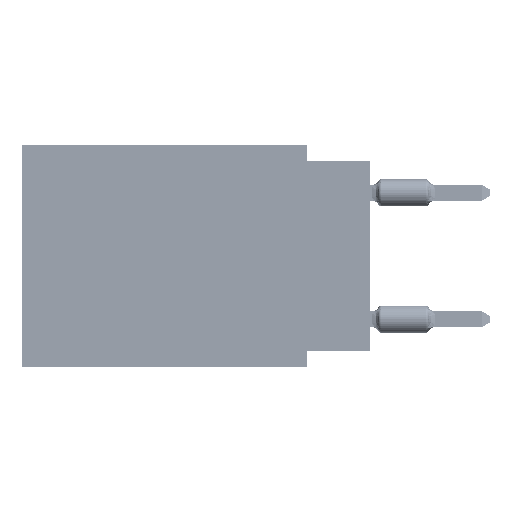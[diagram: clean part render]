
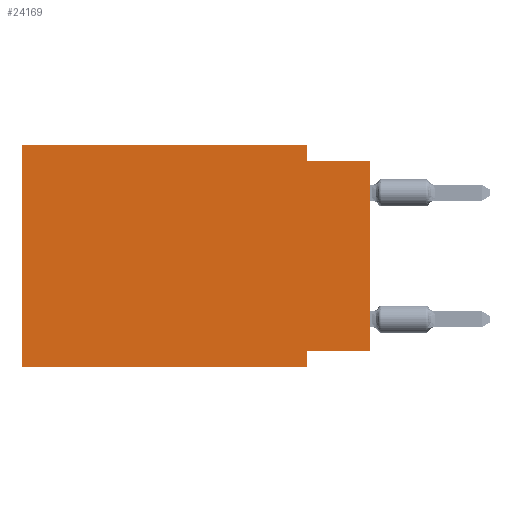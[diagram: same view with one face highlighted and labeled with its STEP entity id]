
A CAD part, left-side view. The second image highlights one B-rep face of the part: STEP entity #24169.
In plain terms, the highlighted planar face has unit normal (-1, 0, 0).
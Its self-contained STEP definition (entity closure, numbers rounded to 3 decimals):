
#1095 = DIRECTION ( 'NONE',  ( 0., 0., -1. ) ) ;
#3180 = CARTESIAN_POINT ( 'NONE',  ( 0., 2.54, 0. ) ) ;
#3432 = DIRECTION ( 'NONE',  ( 0., 0., 1. ) ) ;
#3450 = EDGE_CURVE ( 'NONE', #73395, #56345, #50145, .T. ) ;
#3740 = LINE ( 'NONE', #25478, #61603 ) ;
#6093 = ORIENTED_EDGE ( 'NONE', *, *, #75973, .F. ) ;
#7841 = DIRECTION ( 'NONE',  ( 1., 0., 0. ) ) ;
#11093 = EDGE_CURVE ( 'NONE', #56331, #86210, #3740, .T. ) ;
#12605 = CARTESIAN_POINT ( 'NONE',  ( 0., 0., -0.635 ) ) ;
#15490 = CARTESIAN_POINT ( 'NONE',  ( 0., 2.54, 0. ) ) ;
#16771 = ORIENTED_EDGE ( 'NONE', *, *, #11093, .F. ) ;
#18758 = ORIENTED_EDGE ( 'NONE', *, *, #63439, .F. ) ;
#19653 = LINE ( 'NONE', #64535, #55077 ) ;
#21653 = CARTESIAN_POINT ( 'NONE',  ( 0., 0., -8.255 ) ) ;
#21686 = VERTEX_POINT ( 'NONE', #22330 ) ;
#22330 = CARTESIAN_POINT ( 'NONE',  ( 0., 0., -0.635 ) ) ;
#22955 = LINE ( 'NONE', #95357, #72637 ) ;
#24169 = ADVANCED_FACE ( 'NONE', ( #59992 ), #25060, .F. ) ;
#25060 = PLANE ( 'NONE',  #44140 ) ;
#25478 = CARTESIAN_POINT ( 'NONE',  ( 0., 13.97, 0. ) ) ;
#27427 = VECTOR ( 'NONE', #3432, 1000. ) ;
#29422 = ORIENTED_EDGE ( 'NONE', *, *, #3450, .F. ) ;
#29690 = DIRECTION ( 'NONE',  ( 0., 0., 1. ) ) ;
#31078 = LINE ( 'NONE', #38805, #72762 ) ;
#33893 = VERTEX_POINT ( 'NONE', #85023 ) ;
#34113 = DIRECTION ( 'NONE',  ( 0., -1., 0. ) ) ;
#37399 = VERTEX_POINT ( 'NONE', #93311 ) ;
#37452 = CARTESIAN_POINT ( 'NONE',  ( 0., 13.97, 0. ) ) ;
#38805 = CARTESIAN_POINT ( 'NONE',  ( 0., 2.54, -8.89 ) ) ;
#39951 = VECTOR ( 'NONE', #74400, 1000. ) ;
#40619 = LINE ( 'NONE', #12605, #46738 ) ;
#44140 = AXIS2_PLACEMENT_3D ( 'NONE', #82180, #7841, #1095 ) ;
#45012 = ORIENTED_EDGE ( 'NONE', *, *, #51847, .F. ) ;
#46738 = VECTOR ( 'NONE', #93222, 1000. ) ;
#47497 = EDGE_CURVE ( 'NONE', #92814, #21686, #40619, .T. ) ;
#50145 = LINE ( 'NONE', #21653, #57371 ) ;
#50817 = EDGE_CURVE ( 'NONE', #33893, #37399, #19653, .T. ) ;
#51847 = EDGE_CURVE ( 'NONE', #86210, #92814, #54057, .T. ) ;
#53290 = ORIENTED_EDGE ( 'NONE', *, *, #47497, .F. ) ;
#54057 = LINE ( 'NONE', #15490, #39951 ) ;
#55077 = VECTOR ( 'NONE', #95409, 1000. ) ;
#56331 = VERTEX_POINT ( 'NONE', #37452 ) ;
#56345 = VERTEX_POINT ( 'NONE', #80438 ) ;
#56593 = CARTESIAN_POINT ( 'NONE',  ( 0., 2.54, -0.635 ) ) ;
#57371 = VECTOR ( 'NONE', #66071, 1000. ) ;
#59992 = FACE_OUTER_BOUND ( 'NONE', #76556, .T. ) ;
#61603 = VECTOR ( 'NONE', #34113, 1000. ) ;
#63439 = EDGE_CURVE ( 'NONE', #56345, #37399, #31078, .T. ) ;
#64044 = ORIENTED_EDGE ( 'NONE', *, *, #50817, .T. ) ;
#64535 = CARTESIAN_POINT ( 'NONE',  ( 0., 13.97, -8.89 ) ) ;
#66071 = DIRECTION ( 'NONE',  ( 0., 1., 0. ) ) ;
#70997 = LINE ( 'NONE', #78704, #27427 ) ;
#71255 = ORIENTED_EDGE ( 'NONE', *, *, #74214, .T. ) ;
#72637 = VECTOR ( 'NONE', #29690, 1000. ) ;
#72762 = VECTOR ( 'NONE', #83225, 1000. ) ;
#73395 = VERTEX_POINT ( 'NONE', #79327 ) ;
#74214 = EDGE_CURVE ( 'NONE', #73395, #21686, #22955, .T. ) ;
#74400 = DIRECTION ( 'NONE',  ( 0., 0., -1. ) ) ;
#75973 = EDGE_CURVE ( 'NONE', #33893, #56331, #70997, .T. ) ;
#76556 = EDGE_LOOP ( 'NONE', ( #71255, #53290, #45012, #16771, #6093, #64044, #18758, #29422 ) ) ;
#78704 = CARTESIAN_POINT ( 'NONE',  ( 0., 13.97, 0. ) ) ;
#79327 = CARTESIAN_POINT ( 'NONE',  ( 0., 0., -8.255 ) ) ;
#80438 = CARTESIAN_POINT ( 'NONE',  ( 0., 2.54, -8.255 ) ) ;
#82180 = CARTESIAN_POINT ( 'NONE',  ( 0., 13.97, 0. ) ) ;
#83225 = DIRECTION ( 'NONE',  ( 0., 0., -1. ) ) ;
#85023 = CARTESIAN_POINT ( 'NONE',  ( 0., 13.97, -8.89 ) ) ;
#86210 = VERTEX_POINT ( 'NONE', #3180 ) ;
#92814 = VERTEX_POINT ( 'NONE', #56593 ) ;
#93222 = DIRECTION ( 'NONE',  ( 0., -1., 0. ) ) ;
#93311 = CARTESIAN_POINT ( 'NONE',  ( 0., 2.54, -8.89 ) ) ;
#95357 = CARTESIAN_POINT ( 'NONE',  ( 0., 0., 0. ) ) ;
#95409 = DIRECTION ( 'NONE',  ( 0., -1., 0. ) ) ;
